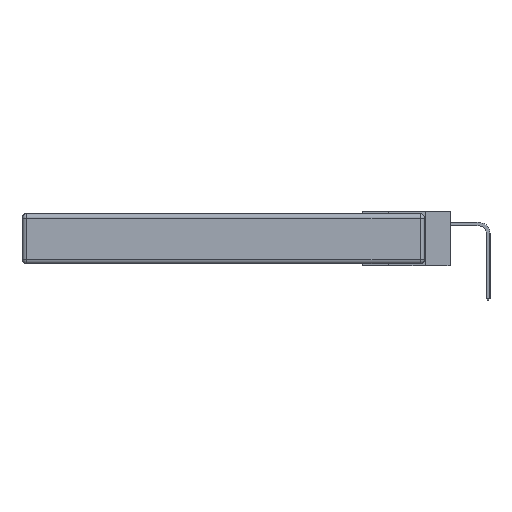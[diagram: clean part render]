
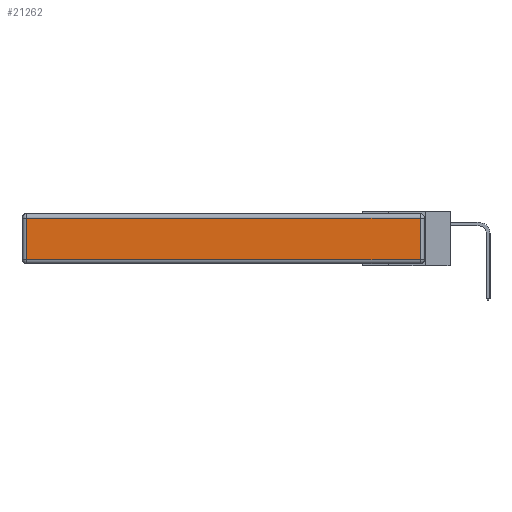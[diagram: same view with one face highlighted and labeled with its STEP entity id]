
A CAD part, left-side view. The second image highlights one B-rep face of the part: STEP entity #21262.
In plain terms, the highlighted planar face has unit normal (-1, 0, 0).
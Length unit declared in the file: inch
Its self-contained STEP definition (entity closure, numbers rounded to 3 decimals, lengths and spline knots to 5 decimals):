
#336 = LINE ( 'NONE', #17982, #17774 ) ;
#1431 = EDGE_LOOP ( 'NONE', ( #14785, #9827, #12819, #13755 ) ) ;
#1909 = VECTOR ( 'NONE', #4294, 39.37008 ) ;
#2096 = CARTESIAN_POINT ( 'NONE',  ( 0., 0., -0.343 ) ) ;
#2121 = AXIS2_PLACEMENT_3D ( 'NONE', #2096, #5588, #5743 ) ;
#2267 = LINE ( 'NONE', #22093, #18930 ) ;
#2552 = CARTESIAN_POINT ( 'NONE',  ( 0., 2.72, -0.343 ) ) ;
#2699 = DIRECTION ( 'NONE',  ( 0., 0., 1. ) ) ;
#3530 = CARTESIAN_POINT ( 'NONE',  ( 0., 2.72, -0.03 ) ) ;
#3858 = LINE ( 'NONE', #11353, #12829 ) ;
#4294 = DIRECTION ( 'NONE',  ( 0., 0., -1. ) ) ;
#5588 = DIRECTION ( 'NONE',  ( -1., 0., 0. ) ) ;
#5743 = DIRECTION ( 'NONE',  ( 0., 0., 1. ) ) ;
#8484 = CARTESIAN_POINT ( 'NONE',  ( 0., 0.03, -0.313 ) ) ;
#8811 = VERTEX_POINT ( 'NONE', #8484 ) ;
#9011 = PLANE ( 'NONE',  #2121 ) ;
#9388 = VERTEX_POINT ( 'NONE', #3530 ) ;
#9827 = ORIENTED_EDGE ( 'NONE', *, *, #13250, .T. ) ;
#9834 = CARTESIAN_POINT ( 'NONE',  ( 0., 2.72, -0.313 ) ) ;
#11139 = LINE ( 'NONE', #2552, #1909 ) ;
#11353 = CARTESIAN_POINT ( 'NONE',  ( 0., 0.03, -0.343 ) ) ;
#12020 = EDGE_CURVE ( 'NONE', #21768, #9388, #2267, .T. ) ;
#12819 = ORIENTED_EDGE ( 'NONE', *, *, #12020, .T. ) ;
#12829 = VECTOR ( 'NONE', #2699, 39.37008 ) ;
#13250 = EDGE_CURVE ( 'NONE', #8811, #21768, #3858, .T. ) ;
#13755 = ORIENTED_EDGE ( 'NONE', *, *, #18060, .T. ) ;
#14785 = ORIENTED_EDGE ( 'NONE', *, *, #16389, .T. ) ;
#16389 = EDGE_CURVE ( 'NONE', #19539, #8811, #336, .T. ) ;
#17555 = FACE_OUTER_BOUND ( 'NONE', #1431, .T. ) ;
#17774 = VECTOR ( 'NONE', #18141, 39.37008 ) ;
#17982 = CARTESIAN_POINT ( 'NONE',  ( 0., 0., -0.313 ) ) ;
#18060 = EDGE_CURVE ( 'NONE', #9388, #19539, #11139, .T. ) ;
#18141 = DIRECTION ( 'NONE',  ( 0., -1., 0. ) ) ;
#18930 = VECTOR ( 'NONE', #21942, 39.37008 ) ;
#19304 = CARTESIAN_POINT ( 'NONE',  ( 0., 0.03, -0.03 ) ) ;
#19539 = VERTEX_POINT ( 'NONE', #9834 ) ;
#21262 = ADVANCED_FACE ( 'NONE', ( #17555 ), #9011, .T. ) ;
#21768 = VERTEX_POINT ( 'NONE', #19304 ) ;
#21942 = DIRECTION ( 'NONE',  ( 0., 1., 0. ) ) ;
#22093 = CARTESIAN_POINT ( 'NONE',  ( 0., 2.75, -0.03 ) ) ;
